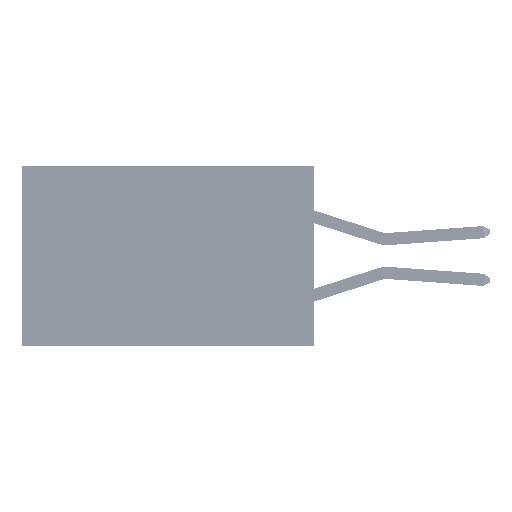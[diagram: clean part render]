
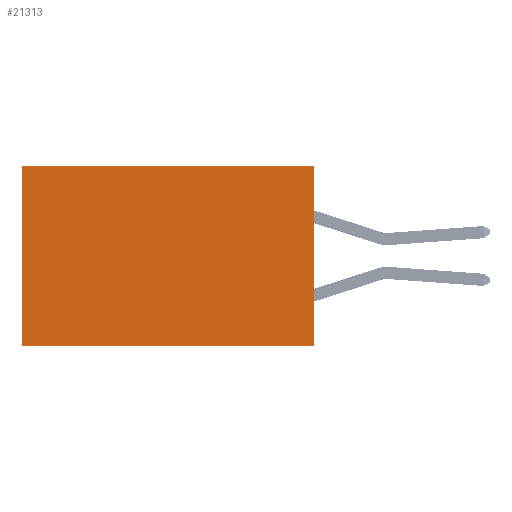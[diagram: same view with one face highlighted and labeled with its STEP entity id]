
A CAD part, left-side view. The second image highlights one B-rep face of the part: STEP entity #21313.
In plain terms, the highlighted planar face has unit normal (-1, 0, 0).
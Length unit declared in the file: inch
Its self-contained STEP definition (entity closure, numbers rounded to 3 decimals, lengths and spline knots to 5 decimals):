
#207 = DIRECTION ( 'NONE',  ( 0., 0., -1. ) ) ;
#1353 = CARTESIAN_POINT ( 'NONE',  ( 0.2875, 0., 0. ) ) ;
#1538 = EDGE_CURVE ( 'NONE', #35164, #10926, #24046, .T. ) ;
#2691 = LINE ( 'NONE', #43905, #32824 ) ;
#3035 = CARTESIAN_POINT ( 'NONE',  ( 0.2875, 0., -0.37 ) ) ;
#3442 = ORIENTED_EDGE ( 'NONE', *, *, #33071, .T. ) ;
#7233 = ORIENTED_EDGE ( 'NONE', *, *, #1538, .F. ) ;
#9138 = LINE ( 'NONE', #1353, #40821 ) ;
#10926 = VERTEX_POINT ( 'NONE', #31689 ) ;
#12194 = VECTOR ( 'NONE', #29276, 39.37008 ) ;
#13550 = CARTESIAN_POINT ( 'NONE',  ( 0.2875, 0., 0. ) ) ;
#13699 = DIRECTION ( 'NONE',  ( 0., 0., -1. ) ) ;
#16236 = EDGE_LOOP ( 'NONE', ( #17754, #7233, #28485, #3442 ) ) ;
#17754 = ORIENTED_EDGE ( 'NONE', *, *, #24502, .T. ) ;
#18373 = VERTEX_POINT ( 'NONE', #32709 ) ;
#20635 = DIRECTION ( 'NONE',  ( 1., 0., 0. ) ) ;
#21313 = ADVANCED_FACE ( 'NONE', ( #31730 ), #33978, .F. ) ;
#24046 = LINE ( 'NONE', #29855, #12194 ) ;
#24502 = EDGE_CURVE ( 'NONE', #41364, #10926, #2691, .T. ) ;
#25258 = CARTESIAN_POINT ( 'NONE',  ( 0.2875, 0.6, 0. ) ) ;
#27738 = CARTESIAN_POINT ( 'NONE',  ( 0.2875, 0., 0. ) ) ;
#28485 = ORIENTED_EDGE ( 'NONE', *, *, #42397, .F. ) ;
#29276 = DIRECTION ( 'NONE',  ( 0., 1., 0. ) ) ;
#29855 = CARTESIAN_POINT ( 'NONE',  ( 0.2875, 0., -0.37 ) ) ;
#31689 = CARTESIAN_POINT ( 'NONE',  ( 0.2875, 0.6, -0.37 ) ) ;
#31730 = FACE_OUTER_BOUND ( 'NONE', #16236, .T. ) ;
#32709 = CARTESIAN_POINT ( 'NONE',  ( 0.2875, 0., 0. ) ) ;
#32824 = VECTOR ( 'NONE', #43450, 39.37008 ) ;
#33071 = EDGE_CURVE ( 'NONE', #18373, #41364, #9138, .T. ) ;
#33978 = PLANE ( 'NONE',  #37923 ) ;
#35164 = VERTEX_POINT ( 'NONE', #3035 ) ;
#35460 = DIRECTION ( 'NONE',  ( 0., 1., 0. ) ) ;
#37923 = AXIS2_PLACEMENT_3D ( 'NONE', #13550, #20635, #13699 ) ;
#40821 = VECTOR ( 'NONE', #35460, 39.37008 ) ;
#41210 = LINE ( 'NONE', #27738, #42310 ) ;
#41364 = VERTEX_POINT ( 'NONE', #25258 ) ;
#42310 = VECTOR ( 'NONE', #207, 39.37008 ) ;
#42397 = EDGE_CURVE ( 'NONE', #18373, #35164, #41210, .T. ) ;
#43450 = DIRECTION ( 'NONE',  ( 0., 0., -1. ) ) ;
#43905 = CARTESIAN_POINT ( 'NONE',  ( 0.2875, 0.6, 0. ) ) ;
